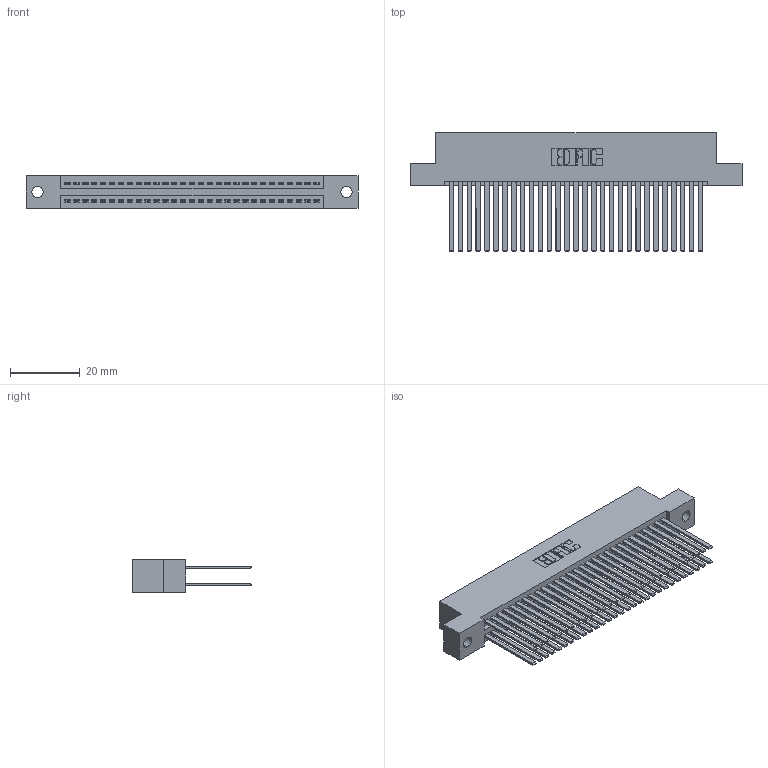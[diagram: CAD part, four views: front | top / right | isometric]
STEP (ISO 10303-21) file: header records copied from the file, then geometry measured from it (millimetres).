
FILE_DESCRIPTION (( 'STEP AP203' ), '1' );
FILE_NAME ('395-058-544-202.STEP', '2019-10-23T12:31:17', ( '' ), ( '' ), 'SwSTEP 2.0', 'SolidWorks 2016', '' );
FILE_SCHEMA (( 'CONFIG_CONTROL_DESIGN' ));
Length unit declared in the file: inch
Products named in the file (3): 345 Part_Flush Mounting Lugs - 0.128 Dia; 345-292-001_345-293-144; 395-058-544-202
Assembly tree (59 placements, depth 2):
  395-058-544-202
    345 Part_Flush Mounting Lugs - 0.128 Dia
    345-292-001_345-293-144  x58
Bounding box: 94.87 x 33.96 x 9.4 mm (x, y, z)
Volume: 9871.4 mm3; surface area: 16450 mm2
Topology: 59 solids, 59 shells, 2678 faces, 7939 edges, 5214 vertices
Faces by surface type: plane 1762, cylinder 916
Entity records: 24323 total; most frequent: CARTESIAN_POINT 4088, ORIENTED_EDGE 4022, DIRECTION 3619, EDGE_CURVE 2011, LINE 1767, VECTOR 1767, VERTEX_POINT 1338, AXIS2_PLACEMENT_3D 926
